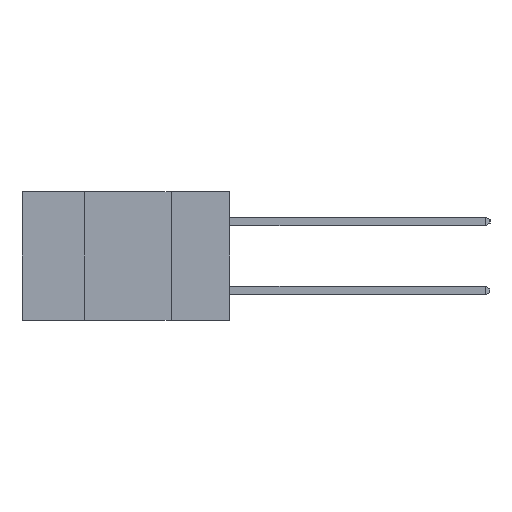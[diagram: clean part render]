
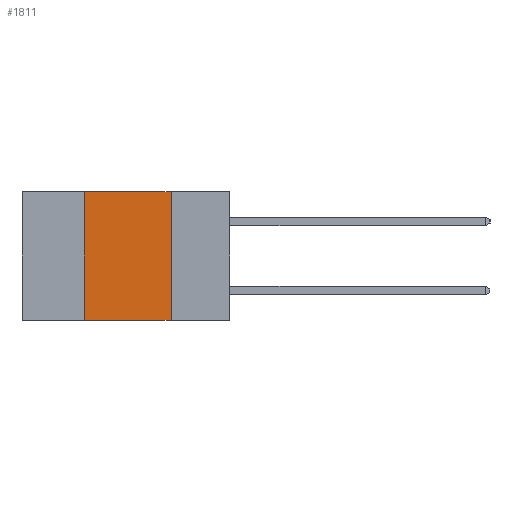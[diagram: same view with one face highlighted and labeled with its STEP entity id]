
A CAD part, left-side view. The second image highlights one B-rep face of the part: STEP entity #1811.
In plain terms, the highlighted planar face has unit normal (-1, 0, 0).
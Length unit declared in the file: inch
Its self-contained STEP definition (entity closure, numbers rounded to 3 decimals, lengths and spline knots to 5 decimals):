
#55 = CARTESIAN_POINT ( 'NONE',  ( 0., 0.42, -0.37 ) ) ;
#155 = CARTESIAN_POINT ( 'NONE',  ( 0., 0.42, 0. ) ) ;
#475 = LINE ( 'NONE', #3361, #2305 ) ;
#525 = EDGE_CURVE ( 'NONE', #4734, #4260, #5299, .T. ) ;
#642 = ORIENTED_EDGE ( 'NONE', *, *, #6566, .F. ) ;
#745 = CARTESIAN_POINT ( 'NONE',  ( 0., 0.6, 0. ) ) ;
#1425 = EDGE_LOOP ( 'NONE', ( #642, #4563, #8657, #1813 ) ) ;
#1490 = LINE ( 'NONE', #2878, #5350 ) ;
#1585 = DIRECTION ( 'NONE',  ( 1., 0., 0. ) ) ;
#1811 = ADVANCED_FACE ( 'NONE', ( #2470 ), #4341, .F. ) ;
#1813 = ORIENTED_EDGE ( 'NONE', *, *, #4146, .T. ) ;
#2305 = VECTOR ( 'NONE', #5323, 39.37008 ) ;
#2469 = DIRECTION ( 'NONE',  ( 0., 0., -1. ) ) ;
#2470 = FACE_OUTER_BOUND ( 'NONE', #1425, .T. ) ;
#2878 = CARTESIAN_POINT ( 'NONE',  ( 0., 0.42, 0. ) ) ;
#3361 = CARTESIAN_POINT ( 'NONE',  ( 0., 0.17, 0. ) ) ;
#4146 = EDGE_CURVE ( 'NONE', #7426, #5162, #8406, .T. ) ;
#4260 = VERTEX_POINT ( 'NONE', #7530 ) ;
#4341 = PLANE ( 'NONE',  #5952 ) ;
#4563 = ORIENTED_EDGE ( 'NONE', *, *, #525, .F. ) ;
#4734 = VERTEX_POINT ( 'NONE', #155 ) ;
#4779 = VECTOR ( 'NONE', #6923, 39.37008 ) ;
#5065 = VECTOR ( 'NONE', #7027, 39.37008 ) ;
#5162 = VERTEX_POINT ( 'NONE', #5341 ) ;
#5195 = EDGE_CURVE ( 'NONE', #7426, #4734, #1490, .T. ) ;
#5299 = LINE ( 'NONE', #745, #5065 ) ;
#5323 = DIRECTION ( 'NONE',  ( 0., 0., -1. ) ) ;
#5341 = CARTESIAN_POINT ( 'NONE',  ( 0., 0.17, -0.37 ) ) ;
#5350 = VECTOR ( 'NONE', #8493, 39.37008 ) ;
#5952 = AXIS2_PLACEMENT_3D ( 'NONE', #8862, #1585, #2469 ) ;
#6566 = EDGE_CURVE ( 'NONE', #4260, #5162, #475, .T. ) ;
#6923 = DIRECTION ( 'NONE',  ( 0., -1., 0. ) ) ;
#7027 = DIRECTION ( 'NONE',  ( 0., -1., 0. ) ) ;
#7426 = VERTEX_POINT ( 'NONE', #55 ) ;
#7530 = CARTESIAN_POINT ( 'NONE',  ( 0., 0.17, 0. ) ) ;
#7984 = CARTESIAN_POINT ( 'NONE',  ( 0., 0.6, -0.37 ) ) ;
#8406 = LINE ( 'NONE', #7984, #4779 ) ;
#8493 = DIRECTION ( 'NONE',  ( 0., 0., 1. ) ) ;
#8657 = ORIENTED_EDGE ( 'NONE', *, *, #5195, .F. ) ;
#8862 = CARTESIAN_POINT ( 'NONE',  ( 0., 0.6, 0. ) ) ;
